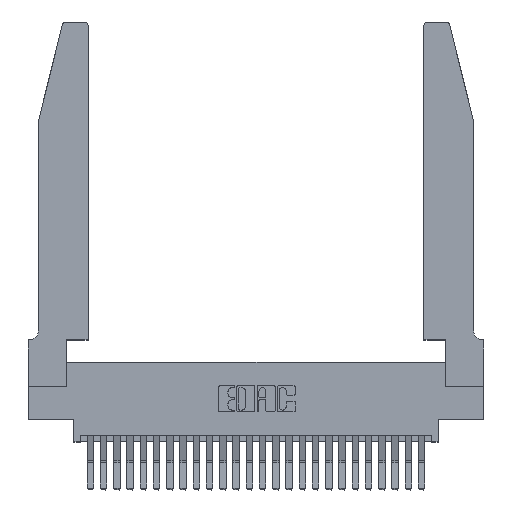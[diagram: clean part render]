
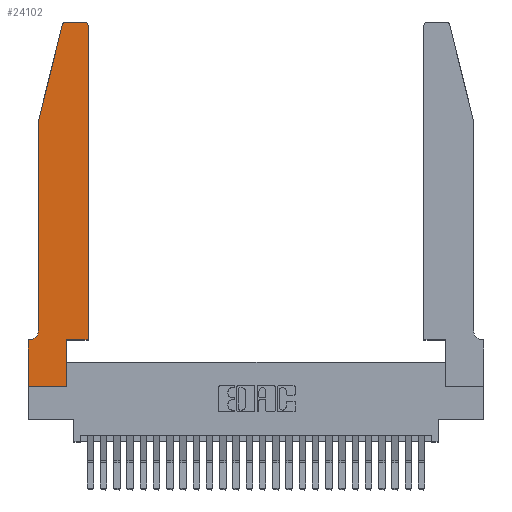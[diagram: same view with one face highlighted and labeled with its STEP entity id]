
A CAD part, top view. The second image highlights one B-rep face of the part: STEP entity #24102.
In plain terms, the highlighted planar face has unit normal (0, 0, 1).
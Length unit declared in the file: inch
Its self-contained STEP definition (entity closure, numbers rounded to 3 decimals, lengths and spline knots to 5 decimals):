
#192 = CARTESIAN_POINT ( 'NONE',  ( 0.2865, 0., 0.37 ) ) ;
#1222 = CARTESIAN_POINT ( 'NONE',  ( 0., 0., 0.37 ) ) ;
#1802 = ORIENTED_EDGE ( 'NONE', *, *, #17397, .T. ) ;
#3110 = EDGE_CURVE ( 'NONE', #25985, #11802, #16802, .T. ) ;
#3177 = VECTOR ( 'NONE', #27052, 39.37008 ) ;
#3598 = DIRECTION ( 'NONE',  ( 0., 1., 0. ) ) ;
#3629 = CARTESIAN_POINT ( 'NONE',  ( 0.4505, 0.35, 0.37 ) ) ;
#4505 = ORIENTED_EDGE ( 'NONE', *, *, #17175, .T. ) ;
#5158 = VERTEX_POINT ( 'NONE', #20559 ) ;
#5187 = DIRECTION ( 'NONE',  ( 0., 0., -1. ) ) ;
#5279 = CARTESIAN_POINT ( 'NONE',  ( 0.284, 2.75, 0.37 ) ) ;
#5335 = LINE ( 'NONE', #10398, #21650 ) ;
#5397 = EDGE_CURVE ( 'NONE', #25587, #5158, #26860, .T. ) ;
#5655 = EDGE_LOOP ( 'NONE', ( #7070, #5767, #9488, #10091, #22967, #27392, #8190, #4505, #23589, #8294, #11017, #1802 ) ) ;
#5767 = ORIENTED_EDGE ( 'NONE', *, *, #8053, .T. ) ;
#6166 = VECTOR ( 'NONE', #23195, 39.37008 ) ;
#6870 = LINE ( 'NONE', #7803, #11267 ) ;
#7070 = ORIENTED_EDGE ( 'NONE', *, *, #14589, .T. ) ;
#7542 = DIRECTION ( 'NONE',  ( 0., 1., 0. ) ) ;
#7803 = CARTESIAN_POINT ( 'NONE',  ( 0.4505, 0.35, 0.37 ) ) ;
#7806 = EDGE_CURVE ( 'NONE', #8660, #26259, #6870, .T. ) ;
#8053 = EDGE_CURVE ( 'NONE', #23707, #25587, #10924, .T. ) ;
#8190 = ORIENTED_EDGE ( 'NONE', *, *, #11088, .T. ) ;
#8294 = ORIENTED_EDGE ( 'NONE', *, *, #25247, .T. ) ;
#8466 = CARTESIAN_POINT ( 'NONE',  ( 0.0755, 2., 0.37 ) ) ;
#8660 = VERTEX_POINT ( 'NONE', #13204 ) ;
#9488 = ORIENTED_EDGE ( 'NONE', *, *, #5397, .T. ) ;
#10091 = ORIENTED_EDGE ( 'NONE', *, *, #17067, .T. ) ;
#10398 = CARTESIAN_POINT ( 'NONE',  ( 0., 0., 0.37 ) ) ;
#10544 = CARTESIAN_POINT ( 'NONE',  ( 0., 0., 0.37 ) ) ;
#10819 = FACE_OUTER_BOUND ( 'NONE', #5655, .T. ) ;
#10829 = CARTESIAN_POINT ( 'NONE',  ( 0.2605, 2.75, 0.37 ) ) ;
#10845 = CARTESIAN_POINT ( 'NONE',  ( 0.284, 2.72, 0.37 ) ) ;
#10917 = DIRECTION ( 'NONE',  ( 1., 0., 0. ) ) ;
#10924 = CIRCLE ( 'NONE', #16568, 0.03 ) ;
#11017 = ORIENTED_EDGE ( 'NONE', *, *, #7806, .T. ) ;
#11088 = EDGE_CURVE ( 'NONE', #11802, #20070, #5335, .T. ) ;
#11267 = VECTOR ( 'NONE', #3598, 39.37008 ) ;
#11369 = DIRECTION ( 'NONE',  ( 0., 0., 1. ) ) ;
#11588 = VECTOR ( 'NONE', #12709, 39.37008 ) ;
#11802 = VERTEX_POINT ( 'NONE', #27322 ) ;
#12012 = VECTOR ( 'NONE', #7542, 39.37008 ) ;
#12517 = AXIS2_PLACEMENT_3D ( 'NONE', #24019, #11369, #26104 ) ;
#12558 = LINE ( 'NONE', #10544, #6166 ) ;
#12709 = DIRECTION ( 'NONE',  ( -1., 0., 0. ) ) ;
#12779 = CARTESIAN_POINT ( 'NONE',  ( 0.0055, 0.35, 0.37 ) ) ;
#12942 = DIRECTION ( 'NONE',  ( 1., 0., 0. ) ) ;
#13204 = CARTESIAN_POINT ( 'NONE',  ( 0.4505, 0.35, 0.37 ) ) ;
#13216 = AXIS2_PLACEMENT_3D ( 'NONE', #21449, #23565, #10917 ) ;
#13865 = LINE ( 'NONE', #10829, #20186 ) ;
#14589 = EDGE_CURVE ( 'NONE', #19353, #23707, #13865, .T. ) ;
#14974 = VECTOR ( 'NONE', #27417, 39.37008 ) ;
#15205 = LINE ( 'NONE', #24941, #3177 ) ;
#15377 = LINE ( 'NONE', #3629, #25915 ) ;
#15793 = VERTEX_POINT ( 'NONE', #192 ) ;
#16568 = AXIS2_PLACEMENT_3D ( 'NONE', #10845, #25575, #12942 ) ;
#16760 = DIRECTION ( 'NONE',  ( 0., -1., 0. ) ) ;
#16802 = LINE ( 'NONE', #23248, #11588 ) ;
#17067 = EDGE_CURVE ( 'NONE', #5158, #25614, #15205, .T. ) ;
#17175 = EDGE_CURVE ( 'NONE', #20070, #15793, #12558, .T. ) ;
#17397 = EDGE_CURVE ( 'NONE', #26259, #19353, #18519, .T. ) ;
#17553 = CARTESIAN_POINT ( 'NONE',  ( 0.2865, 0.35, 0.37 ) ) ;
#17617 = CARTESIAN_POINT ( 'NONE',  ( 0.25487, 2.72718, 0.37 ) ) ;
#17958 = CARTESIAN_POINT ( 'NONE',  ( 0.0055, 0.42, 0.37 ) ) ;
#18519 = CIRCLE ( 'NONE', #12517, 0.03 ) ;
#19340 = PLANE ( 'NONE',  #13216 ) ;
#19353 = VERTEX_POINT ( 'NONE', #23723 ) ;
#20070 = VERTEX_POINT ( 'NONE', #1222 ) ;
#20107 = DIRECTION ( 'NONE',  ( -1., 0., 0. ) ) ;
#20186 = VECTOR ( 'NONE', #25557, 39.37008 ) ;
#20559 = CARTESIAN_POINT ( 'NONE',  ( 0.0755, 2., 0.37 ) ) ;
#20694 = DIRECTION ( 'NONE',  ( 1., 0., 0. ) ) ;
#21246 = EDGE_CURVE ( 'NONE', #15793, #24993, #23244, .T. ) ;
#21449 = CARTESIAN_POINT ( 'NONE',  ( 0., 0.35, 0.37 ) ) ;
#21650 = VECTOR ( 'NONE', #16760, 39.37008 ) ;
#22967 = ORIENTED_EDGE ( 'NONE', *, *, #26183, .T. ) ;
#23195 = DIRECTION ( 'NONE',  ( 1., 0., 0. ) ) ;
#23244 = LINE ( 'NONE', #24533, #12012 ) ;
#23248 = CARTESIAN_POINT ( 'NONE',  ( 0.0755, 0.35, 0.37 ) ) ;
#23342 = AXIS2_PLACEMENT_3D ( 'NONE', #17958, #5187, #20107 ) ;
#23565 = DIRECTION ( 'NONE',  ( 0., 0., 1. ) ) ;
#23589 = ORIENTED_EDGE ( 'NONE', *, *, #21246, .T. ) ;
#23707 = VERTEX_POINT ( 'NONE', #5279 ) ;
#23723 = CARTESIAN_POINT ( 'NONE',  ( 0.4205, 2.75, 0.37 ) ) ;
#24019 = CARTESIAN_POINT ( 'NONE',  ( 0.4205, 2.72, 0.37 ) ) ;
#24102 = ADVANCED_FACE ( 'NONE', ( #10819 ), #19340, .T. ) ;
#24403 = CARTESIAN_POINT ( 'NONE',  ( 0.4505, 2.72, 0.37 ) ) ;
#24533 = CARTESIAN_POINT ( 'NONE',  ( 0.2865, 0.35, 0.37 ) ) ;
#24941 = CARTESIAN_POINT ( 'NONE',  ( 0.0755, 2., 0.37 ) ) ;
#24993 = VERTEX_POINT ( 'NONE', #17553 ) ;
#25247 = EDGE_CURVE ( 'NONE', #24993, #8660, #15377, .T. ) ;
#25557 = DIRECTION ( 'NONE',  ( -1., 0., 0. ) ) ;
#25575 = DIRECTION ( 'NONE',  ( 0., 0., 1. ) ) ;
#25587 = VERTEX_POINT ( 'NONE', #17617 ) ;
#25614 = VERTEX_POINT ( 'NONE', #26162 ) ;
#25915 = VECTOR ( 'NONE', #20694, 39.37008 ) ;
#25985 = VERTEX_POINT ( 'NONE', #12779 ) ;
#26104 = DIRECTION ( 'NONE',  ( 1., 0., 0. ) ) ;
#26162 = CARTESIAN_POINT ( 'NONE',  ( 0.0755, 0.42, 0.37 ) ) ;
#26183 = EDGE_CURVE ( 'NONE', #25614, #25985, #26248, .T. ) ;
#26248 = CIRCLE ( 'NONE', #23342, 0.07 ) ;
#26259 = VERTEX_POINT ( 'NONE', #24403 ) ;
#26860 = LINE ( 'NONE', #8466, #14974 ) ;
#27052 = DIRECTION ( 'NONE',  ( 0., -1., 0. ) ) ;
#27322 = CARTESIAN_POINT ( 'NONE',  ( 0., 0.35, 0.37 ) ) ;
#27392 = ORIENTED_EDGE ( 'NONE', *, *, #3110, .T. ) ;
#27417 = DIRECTION ( 'NONE',  ( -0.239, -0.971, 0. ) ) ;
